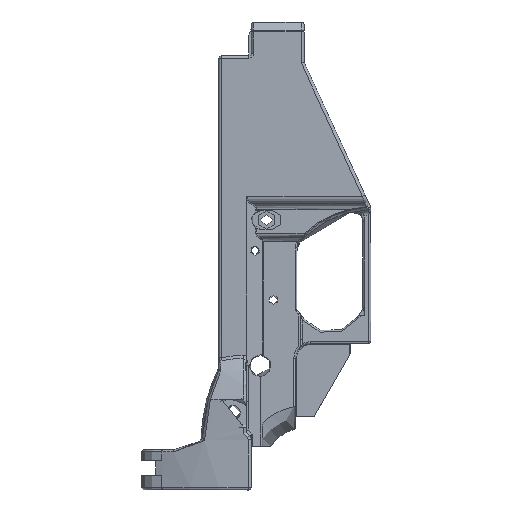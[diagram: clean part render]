
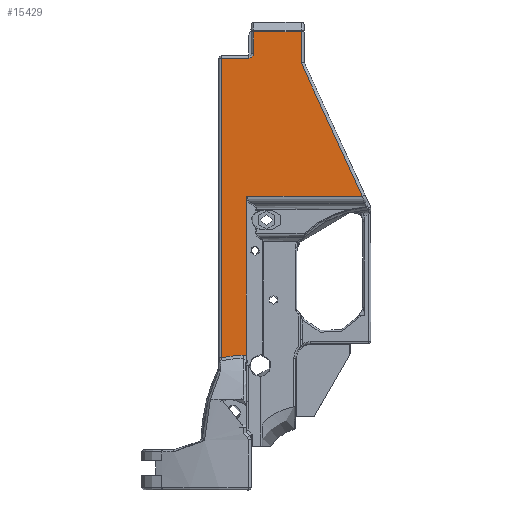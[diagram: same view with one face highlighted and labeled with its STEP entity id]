
A CAD part, left-side view. The second image highlights one B-rep face of the part: STEP entity #15429.
In plain terms, the highlighted planar face has unit normal (-1, 0, 0).
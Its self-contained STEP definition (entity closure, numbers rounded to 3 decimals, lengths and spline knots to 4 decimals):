
#221=ELLIPSE('',#16812,1.9201,1.636);
#396=PLANE('',#16810);
#1332=FACE_OUTER_BOUND('',#2279,.T.);
#2279=EDGE_LOOP('',(#12417,#12418,#12419,#12420,#12421,#12422,#12423,#12424,
#12425,#12426,#12427,#12428));
#3229=B_SPLINE_CURVE_WITH_KNOTS('',3,(#43292,#43293,#43294,#43295),
 .UNSPECIFIED.,.F.,.F.,(4,4),(-0.1434,0.),
 .UNSPECIFIED.);
#3230=B_SPLINE_CURVE_WITH_KNOTS('',3,(#43299,#43300,#43301,#43302,#43303,
#43304,#43305,#43306,#43307,#43308,#43309,#43310),.UNSPECIFIED.,.F.,.F.,
(4,2,2,2,2,4),(-0.117,-0.1147,-0.0798,
-0.057,-0.0072,0.),.UNSPECIFIED.);
#3848=CIRCLE('',#16811,0.08);
#4485=LINE('',#25828,#5254);
#4487=LINE('',#25859,#5256);
#4667=LINE('',#43244,#5436);
#4671=LINE('',#43282,#5440);
#4672=LINE('',#43286,#5441);
#4673=LINE('',#43288,#5442);
#4674=LINE('',#43297,#5443);
#4675=LINE('',#43311,#5444);
#5254=VECTOR('',#19010,0.3937);
#5256=VECTOR('',#19022,0.3937);
#5436=VECTOR('',#19846,0.3937);
#5440=VECTOR('',#19868,0.3937);
#5441=VECTOR('',#19871,0.3937);
#5442=VECTOR('',#19872,0.3937);
#5443=VECTOR('',#19875,1.6985);
#5444=VECTOR('',#19876,0.1181);
#6262=VERTEX_POINT('',#25825);
#6263=VERTEX_POINT('',#25827);
#6267=VERTEX_POINT('',#25857);
#6767=VERTEX_POINT('',#43242);
#6772=VERTEX_POINT('',#43281);
#6773=VERTEX_POINT('',#43283);
#6774=VERTEX_POINT('',#43285);
#6775=VERTEX_POINT('',#43287);
#6776=VERTEX_POINT('',#43289);
#6777=VERTEX_POINT('',#43291);
#6778=VERTEX_POINT('',#43296);
#6779=VERTEX_POINT('',#43298);
#8038=EDGE_CURVE('',#6262,#6263,#4485,.T.);
#8045=EDGE_CURVE('',#6267,#6262,#4487,.T.);
#8778=EDGE_CURVE('',#6767,#6267,#4667,.T.);
#8787=EDGE_CURVE('',#6772,#6767,#4671,.T.);
#8788=EDGE_CURVE('',#6773,#6772,#3848,.T.);
#8789=EDGE_CURVE('',#6774,#6773,#4672,.T.);
#8790=EDGE_CURVE('',#6775,#6774,#4673,.T.);
#8791=EDGE_CURVE('',#6776,#6775,#221,.T.);
#8792=EDGE_CURVE('',#6777,#6776,#3229,.T.);
#8793=EDGE_CURVE('',#6778,#6777,#4674,.T.);
#8794=EDGE_CURVE('',#6779,#6778,#3230,.T.);
#8795=EDGE_CURVE('',#6263,#6779,#4675,.T.);
#12417=ORIENTED_EDGE('',*,*,#8038,.F.);
#12418=ORIENTED_EDGE('',*,*,#8045,.F.);
#12419=ORIENTED_EDGE('',*,*,#8778,.F.);
#12420=ORIENTED_EDGE('',*,*,#8787,.F.);
#12421=ORIENTED_EDGE('',*,*,#8788,.F.);
#12422=ORIENTED_EDGE('',*,*,#8789,.F.);
#12423=ORIENTED_EDGE('',*,*,#8790,.F.);
#12424=ORIENTED_EDGE('',*,*,#8791,.F.);
#12425=ORIENTED_EDGE('',*,*,#8792,.F.);
#12426=ORIENTED_EDGE('',*,*,#8793,.F.);
#12427=ORIENTED_EDGE('',*,*,#8794,.F.);
#12428=ORIENTED_EDGE('',*,*,#8795,.F.);
#15429=ADVANCED_FACE('',(#1332),#396,.F.);
#16810=AXIS2_PLACEMENT_3D('',#43280,#19866,#19867);
#16811=AXIS2_PLACEMENT_3D('',#43284,#19869,#19870);
#16812=AXIS2_PLACEMENT_3D('',#43290,#19873,#19874);
#19010=DIRECTION('',(0.,-0.417,-0.909));
#19022=DIRECTION('',(0.,0.,-1.));
#19846=DIRECTION('',(0.,-1.,0.));
#19866=DIRECTION('center_axis',(1.,0.,0.));
#19867=DIRECTION('ref_axis',(0.,0.,
-1.));
#19868=DIRECTION('',(0.,0.,1.));
#19869=DIRECTION('center_axis',(-1.,0.,0.));
#19870=DIRECTION('ref_axis',(0.,-0.707,-0.707));
#19871=DIRECTION('',(0.,-1.,0.));
#19872=DIRECTION('',(0.,0.,1.));
#19873=DIRECTION('center_axis',(-1.,0.,0.));
#19874=DIRECTION('ref_axis',(0.,-0.984,-0.179));
#19875=DIRECTION('',(0.,0.,-1.));
#19876=DIRECTION('',(0.,1.,0.));
#25825=CARTESIAN_POINT('',(-0.731,-0.0727,2.8507));
#25827=CARTESIAN_POINT('',(-0.731,-1.118,0.5717));
#25828=CARTESIAN_POINT('',(-0.731,-1.4648,-0.1846));
#25857=CARTESIAN_POINT('',(-0.731,-0.0728,3.3816));
#25859=CARTESIAN_POINT('',(-0.731,-0.0727,-0.2092));
#43242=CARTESIAN_POINT('',(-0.731,0.7372,3.3816));
#43244=CARTESIAN_POINT('',(-0.731,0.7121,3.3816));
#43280=CARTESIAN_POINT('Origin',(-0.731,0.68,-3.6849));
#43281=CARTESIAN_POINT('',(-0.731,0.7373,3.0095));
#43282=CARTESIAN_POINT('',(-0.731,0.7373,-0.0118));
#43283=CARTESIAN_POINT('',(-0.731,0.8173,2.9295));
#43284=CARTESIAN_POINT('Origin',(-0.731,0.8173,3.0095));
#43285=CARTESIAN_POINT('',(-0.731,1.2902,2.9295));
#43286=CARTESIAN_POINT('',(-0.731,0.7441,2.9295));
#43287=CARTESIAN_POINT('',(-0.731,1.2902,-2.1813));
#43288=CARTESIAN_POINT('',(-0.731,1.2902,-3.1756));
#43289=CARTESIAN_POINT('',(-0.731,0.9158,-2.1342));
#43290=CARTESIAN_POINT('Origin',(-0.731,0.7244,-3.7785));
#43291=CARTESIAN_POINT('',(-0.731,0.8628,-2.151));
#43292=CARTESIAN_POINT('Ctrl Pts',(-0.731,0.8629,
-2.151));
#43293=CARTESIAN_POINT('Ctrl Pts',(-0.731,0.8784,
-2.1404));
#43294=CARTESIAN_POINT('Ctrl Pts',(-0.731,0.8969,
-2.1335));
#43295=CARTESIAN_POINT('Ctrl Pts',(-0.731,0.9158,
-2.1342));
#43296=CARTESIAN_POINT('',(-0.731,0.8628,0.5319));
#43297=CARTESIAN_POINT('',(-0.731,0.8628,-2.5001));
#43298=CARTESIAN_POINT('',(-0.731,0.8546,0.5717));
#43299=CARTESIAN_POINT('Ctrl Pts',(-0.731,0.8546,
0.5717));
#43300=CARTESIAN_POINT('Ctrl Pts',(-0.731,0.8546,
0.5716));
#43301=CARTESIAN_POINT('Ctrl Pts',(-0.731,0.8546,
0.5716));
#43302=CARTESIAN_POINT('Ctrl Pts',(-0.731,0.855,
0.5706));
#43303=CARTESIAN_POINT('Ctrl Pts',(-0.731,0.8564,
0.5674));
#43304=CARTESIAN_POINT('Ctrl Pts',(-0.731,0.8587,
0.5601));
#43305=CARTESIAN_POINT('Ctrl Pts',(-0.731,0.8595,
0.5572));
#43306=CARTESIAN_POINT('Ctrl Pts',(-0.731,0.8617,
0.5478));
#43307=CARTESIAN_POINT('Ctrl Pts',(-0.731,0.8626,
0.5413));
#43308=CARTESIAN_POINT('Ctrl Pts',(-0.731,0.8628,
0.5338));
#43309=CARTESIAN_POINT('Ctrl Pts',(-0.731,0.8628,
0.5329));
#43310=CARTESIAN_POINT('Ctrl Pts',(-0.731,0.8628,
0.5319));
#43311=CARTESIAN_POINT('',(-0.731,1.0895,0.5717));
